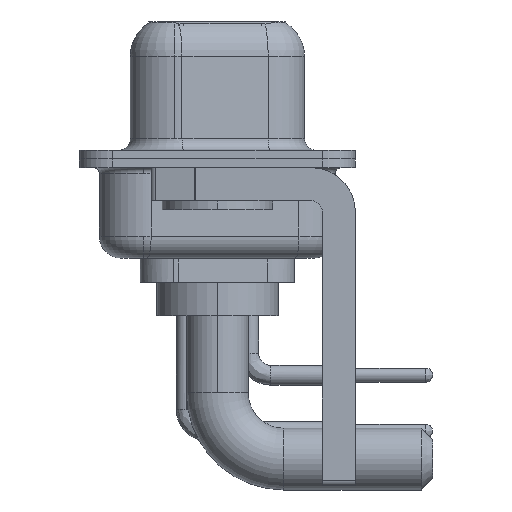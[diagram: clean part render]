
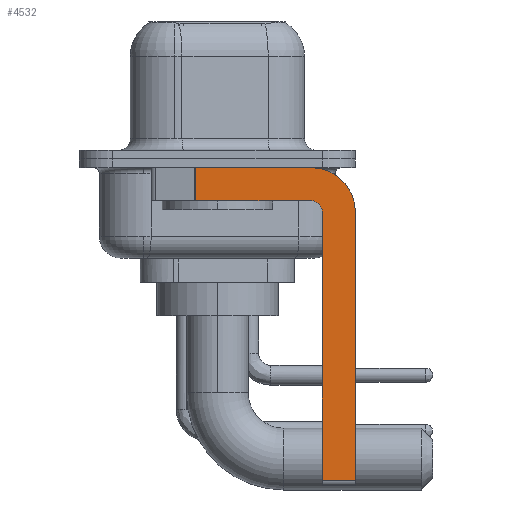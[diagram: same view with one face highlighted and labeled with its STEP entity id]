
A CAD part, left-side view. The second image highlights one B-rep face of the part: STEP entity #4532.
In plain terms, the highlighted planar face has unit normal (-1, 0, 0).
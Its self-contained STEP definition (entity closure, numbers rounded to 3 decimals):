
#98 = EDGE_LOOP ( 'NONE', ( #15984, #8275, #1386, #1980, #885, #7741, #10264, #15223 ) ) ;
#725 = VERTEX_POINT ( 'NONE', #2017 ) ;
#885 = ORIENTED_EDGE ( 'NONE', *, *, #15325, .F. ) ;
#1386 = ORIENTED_EDGE ( 'NONE', *, *, #16183, .F. ) ;
#1487 = LINE ( 'NONE', #17393, #12290 ) ;
#1693 = LINE ( 'NONE', #8669, #7144 ) ;
#1980 = ORIENTED_EDGE ( 'NONE', *, *, #10552, .F. ) ;
#2017 = CARTESIAN_POINT ( 'NONE',  ( -2.9, 0.978, -1.9 ) ) ;
#2573 = CARTESIAN_POINT ( 'NONE',  ( -2.9, -4.25, -2.4 ) ) ;
#2787 = CARTESIAN_POINT ( 'NONE',  ( -2.9, -4.25, -14.55 ) ) ;
#3085 = AXIS2_PLACEMENT_3D ( 'NONE', #2573, #5242, #9285 ) ;
#3267 = CARTESIAN_POINT ( 'NONE',  ( -2.9, -4.75, -2.4 ) ) ;
#3738 = CARTESIAN_POINT ( 'NONE',  ( -2.9, -4.25, -0.4 ) ) ;
#3826 = CARTESIAN_POINT ( 'NONE',  ( -2.9, -4.25, -1.9 ) ) ;
#4025 = DIRECTION ( 'NONE',  ( 0., -1., 0. ) ) ;
#4162 = VERTEX_POINT ( 'NONE', #3826 ) ;
#4532 = ADVANCED_FACE ( 'NONE', ( #9646 ), #13395, .F. ) ;
#4648 = LINE ( 'NONE', #5732, #14219 ) ;
#4795 = EDGE_CURVE ( 'NONE', #10519, #9826, #13108, .T. ) ;
#4909 = VERTEX_POINT ( 'NONE', #3267 ) ;
#5224 = CARTESIAN_POINT ( 'NONE',  ( -2.9, -4.25, -2.4 ) ) ;
#5242 = DIRECTION ( 'NONE',  ( 1., 0., 0. ) ) ;
#5247 = CIRCLE ( 'NONE', #9560, 2. ) ;
#5523 = VERTEX_POINT ( 'NONE', #13530 ) ;
#5732 = CARTESIAN_POINT ( 'NONE',  ( -2.9, -6.25, -2.4 ) ) ;
#5994 = DIRECTION ( 'NONE',  ( 1., 0., 0. ) ) ;
#6390 = CARTESIAN_POINT ( 'NONE',  ( -2.9, 3., -0.4 ) ) ;
#6576 = VECTOR ( 'NONE', #17667, 1000. ) ;
#6847 = VECTOR ( 'NONE', #11698, 1000. ) ;
#6986 = LINE ( 'NONE', #2787, #13130 ) ;
#7144 = VECTOR ( 'NONE', #14109, 1000. ) ;
#7741 = ORIENTED_EDGE ( 'NONE', *, *, #15699, .T. ) ;
#8275 = ORIENTED_EDGE ( 'NONE', *, *, #16500, .T. ) ;
#8669 = CARTESIAN_POINT ( 'NONE',  ( -2.9, -4.25, -1.9 ) ) ;
#8846 = EDGE_CURVE ( 'NONE', #9826, #14784, #5247, .T. ) ;
#8873 = CARTESIAN_POINT ( 'NONE',  ( -2.9, -4.25, -2.4 ) ) ;
#9285 = DIRECTION ( 'NONE',  ( 0., 0., -1. ) ) ;
#9388 = CARTESIAN_POINT ( 'NONE',  ( -2.9, -6.25, -2.4 ) ) ;
#9560 = AXIS2_PLACEMENT_3D ( 'NONE', #8873, #5994, #12974 ) ;
#9639 = CARTESIAN_POINT ( 'NONE',  ( -2.9, 0.978, -1.9 ) ) ;
#9646 = FACE_OUTER_BOUND ( 'NONE', #98, .T. ) ;
#9744 = VERTEX_POINT ( 'NONE', #17339 ) ;
#9826 = VERTEX_POINT ( 'NONE', #3738 ) ;
#10264 = ORIENTED_EDGE ( 'NONE', *, *, #12345, .F. ) ;
#10519 = VERTEX_POINT ( 'NONE', #15693 ) ;
#10552 = EDGE_CURVE ( 'NONE', #4909, #4162, #11613, .T. ) ;
#10623 = DIRECTION ( 'NONE',  ( 0., 0., 1. ) ) ;
#10754 = AXIS2_PLACEMENT_3D ( 'NONE', #5224, #16140, #17121 ) ;
#11221 = DIRECTION ( 'NONE',  ( 0., 0., -1. ) ) ;
#11613 = CIRCLE ( 'NONE', #10754, 0.5 ) ;
#11698 = DIRECTION ( 'NONE',  ( 0., -1., 0. ) ) ;
#12290 = VECTOR ( 'NONE', #10623, 1000. ) ;
#12345 = EDGE_CURVE ( 'NONE', #14784, #5523, #4648, .T. ) ;
#12974 = DIRECTION ( 'NONE',  ( 0., 0., -1. ) ) ;
#13108 = LINE ( 'NONE', #6390, #6847 ) ;
#13130 = VECTOR ( 'NONE', #4025, 1000. ) ;
#13395 = PLANE ( 'NONE',  #3085 ) ;
#13530 = CARTESIAN_POINT ( 'NONE',  ( -2.9, -6.25, -14.55 ) ) ;
#14109 = DIRECTION ( 'NONE',  ( 0., 1., 0. ) ) ;
#14219 = VECTOR ( 'NONE', #11221, 1000. ) ;
#14784 = VERTEX_POINT ( 'NONE', #9388 ) ;
#15223 = ORIENTED_EDGE ( 'NONE', *, *, #8846, .F. ) ;
#15325 = EDGE_CURVE ( 'NONE', #9744, #4909, #1487, .T. ) ;
#15693 = CARTESIAN_POINT ( 'NONE',  ( -2.9, 0.978, -0.4 ) ) ;
#15699 = EDGE_CURVE ( 'NONE', #9744, #5523, #6986, .T. ) ;
#15984 = ORIENTED_EDGE ( 'NONE', *, *, #4795, .F. ) ;
#16140 = DIRECTION ( 'NONE',  ( -1., 0., 0. ) ) ;
#16183 = EDGE_CURVE ( 'NONE', #4162, #725, #1693, .T. ) ;
#16500 = EDGE_CURVE ( 'NONE', #10519, #725, #16508, .T. ) ;
#16508 = LINE ( 'NONE', #9639, #6576 ) ;
#17121 = DIRECTION ( 'NONE',  ( 0., 0., 1. ) ) ;
#17339 = CARTESIAN_POINT ( 'NONE',  ( -2.9, -4.75, -14.55 ) ) ;
#17393 = CARTESIAN_POINT ( 'NONE',  ( -2.9, -4.75, -14.8 ) ) ;
#17667 = DIRECTION ( 'NONE',  ( 0., 0., -1. ) ) ;
